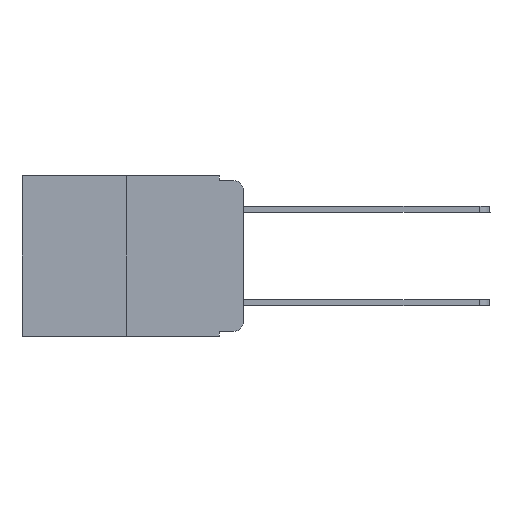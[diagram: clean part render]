
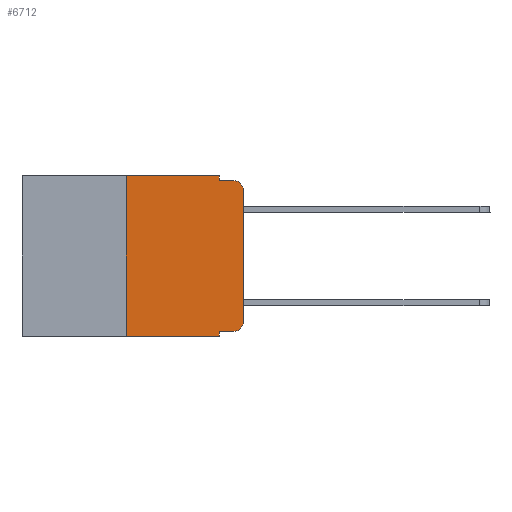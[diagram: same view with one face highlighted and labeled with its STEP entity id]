
A CAD part, left-side view. The second image highlights one B-rep face of the part: STEP entity #6712.
In plain terms, the highlighted planar face has unit normal (-1, 0, 0).
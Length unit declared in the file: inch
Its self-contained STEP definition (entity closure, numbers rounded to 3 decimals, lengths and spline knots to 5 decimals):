
#843 = CARTESIAN_POINT ( 'NONE',  ( 0., 0.25, 0. ) ) ;
#1260 = VECTOR ( 'NONE', #4064, 39.37008 ) ;
#1312 = EDGE_CURVE ( 'NONE', #12646, #7196, #3937, .T. ) ;
#1598 = VECTOR ( 'NONE', #12709, 39.37008 ) ;
#2054 = EDGE_CURVE ( 'NONE', #21031, #15024, #6625, .T. ) ;
#2559 = CARTESIAN_POINT ( 'NONE',  ( 0., 0., -0.03 ) ) ;
#2595 = DIRECTION ( 'NONE',  ( 0., -1., 0. ) ) ;
#2794 = CARTESIAN_POINT ( 'NONE',  ( 0., 0., -0.313 ) ) ;
#3937 = CIRCLE ( 'NONE', #12800, 0.02 ) ;
#4064 = DIRECTION ( 'NONE',  ( 0., -1., 0. ) ) ;
#4126 = ORIENTED_EDGE ( 'NONE', *, *, #8043, .F. ) ;
#4310 = CARTESIAN_POINT ( 'NONE',  ( 0., 0.473, -0.343 ) ) ;
#4584 = VECTOR ( 'NONE', #9415, 39.37008 ) ;
#4660 = DIRECTION ( 'NONE',  ( 0., 0., -1. ) ) ;
#5222 = VERTEX_POINT ( 'NONE', #8206 ) ;
#5336 = VERTEX_POINT ( 'NONE', #10195 ) ;
#5356 = CIRCLE ( 'NONE', #5933, 0.02 ) ;
#5597 = LINE ( 'NONE', #19737, #15118 ) ;
#5824 = DIRECTION ( 'NONE',  ( -1., 0., 0. ) ) ;
#5933 = AXIS2_PLACEMENT_3D ( 'NONE', #21638, #6544, #6464 ) ;
#6302 = DIRECTION ( 'NONE',  ( 1., 0., 0. ) ) ;
#6464 = DIRECTION ( 'NONE',  ( 0., 0., -1. ) ) ;
#6544 = DIRECTION ( 'NONE',  ( -1., 0., 0. ) ) ;
#6625 = LINE ( 'NONE', #4310, #1260 ) ;
#6712 = ADVANCED_FACE ( 'NONE', ( #19662 ), #16188, .F. ) ;
#7117 = CARTESIAN_POINT ( 'NONE',  ( 0., 0.051, -0.01 ) ) ;
#7196 = VERTEX_POINT ( 'NONE', #2794 ) ;
#7393 = VERTEX_POINT ( 'NONE', #14251 ) ;
#7442 = ORIENTED_EDGE ( 'NONE', *, *, #8073, .T. ) ;
#7479 = EDGE_CURVE ( 'NONE', #21050, #5336, #5356, .T. ) ;
#7621 = CARTESIAN_POINT ( 'NONE',  ( 0., 0.051, -0.343 ) ) ;
#7656 = VERTEX_POINT ( 'NONE', #8365 ) ;
#7919 = VECTOR ( 'NONE', #15021, 39.37008 ) ;
#8043 = EDGE_CURVE ( 'NONE', #7656, #5222, #5597, .T. ) ;
#8073 = EDGE_CURVE ( 'NONE', #7393, #12646, #20182, .T. ) ;
#8206 = CARTESIAN_POINT ( 'NONE',  ( 0., 0.051, 0. ) ) ;
#8312 = ORIENTED_EDGE ( 'NONE', *, *, #18660, .F. ) ;
#8330 = EDGE_LOOP ( 'NONE', ( #12256, #11227, #17457, #13143, #4126, #8312, #16956, #19494, #7442, #10292 ) ) ;
#8365 = CARTESIAN_POINT ( 'NONE',  ( 0., 0.25, 0. ) ) ;
#8515 = CARTESIAN_POINT ( 'NONE',  ( 0., 0.051, -0.01 ) ) ;
#9227 = VERTEX_POINT ( 'NONE', #7117 ) ;
#9415 = DIRECTION ( 'NONE',  ( 0., 0., 1. ) ) ;
#10195 = CARTESIAN_POINT ( 'NONE',  ( 0., 0.02, -0.01 ) ) ;
#10292 = ORIENTED_EDGE ( 'NONE', *, *, #1312, .T. ) ;
#11227 = ORIENTED_EDGE ( 'NONE', *, *, #7479, .T. ) ;
#12065 = CARTESIAN_POINT ( 'NONE',  ( 0., 0.051, 0. ) ) ;
#12256 = ORIENTED_EDGE ( 'NONE', *, *, #17833, .T. ) ;
#12416 = LINE ( 'NONE', #8515, #7919 ) ;
#12646 = VERTEX_POINT ( 'NONE', #16381 ) ;
#12709 = DIRECTION ( 'NONE',  ( 0., 0., -1. ) ) ;
#12794 = DIRECTION ( 'NONE',  ( 0., 0., 1. ) ) ;
#12800 = AXIS2_PLACEMENT_3D ( 'NONE', #16087, #5824, #20614 ) ;
#12853 = CARTESIAN_POINT ( 'NONE',  ( 0., 0.051, -0.333 ) ) ;
#12950 = CARTESIAN_POINT ( 'NONE',  ( 0., 0.473, 0. ) ) ;
#13143 = ORIENTED_EDGE ( 'NONE', *, *, #20879, .F. ) ;
#13260 = EDGE_CURVE ( 'NONE', #7393, #15024, #20209, .T. ) ;
#13572 = LINE ( 'NONE', #843, #4584 ) ;
#13980 = CARTESIAN_POINT ( 'NONE',  ( 0., 0., 0. ) ) ;
#14251 = CARTESIAN_POINT ( 'NONE',  ( 0., 0.051, -0.333 ) ) ;
#14387 = CARTESIAN_POINT ( 'NONE',  ( 0., 0.051, 0. ) ) ;
#15021 = DIRECTION ( 'NONE',  ( 0., -1., 0. ) ) ;
#15024 = VERTEX_POINT ( 'NONE', #7621 ) ;
#15118 = VECTOR ( 'NONE', #21387, 39.37008 ) ;
#15380 = DIRECTION ( 'NONE',  ( 0., 0., -1. ) ) ;
#16087 = CARTESIAN_POINT ( 'NONE',  ( 0., 0.02, -0.313 ) ) ;
#16188 = PLANE ( 'NONE',  #19667 ) ;
#16381 = CARTESIAN_POINT ( 'NONE',  ( 0., 0.02, -0.333 ) ) ;
#16956 = ORIENTED_EDGE ( 'NONE', *, *, #2054, .T. ) ;
#17070 = VECTOR ( 'NONE', #12794, 39.37008 ) ;
#17195 = VECTOR ( 'NONE', #15380, 39.37008 ) ;
#17457 = ORIENTED_EDGE ( 'NONE', *, *, #20707, .F. ) ;
#17833 = EDGE_CURVE ( 'NONE', #7196, #21050, #19985, .T. ) ;
#18660 = EDGE_CURVE ( 'NONE', #21031, #7656, #13572, .T. ) ;
#19295 = LINE ( 'NONE', #12065, #17195 ) ;
#19494 = ORIENTED_EDGE ( 'NONE', *, *, #13260, .F. ) ;
#19651 = CARTESIAN_POINT ( 'NONE',  ( 0., 0.25, -0.343 ) ) ;
#19662 = FACE_OUTER_BOUND ( 'NONE', #8330, .T. ) ;
#19667 = AXIS2_PLACEMENT_3D ( 'NONE', #12950, #6302, #4660 ) ;
#19737 = CARTESIAN_POINT ( 'NONE',  ( 0., 0.473, 0. ) ) ;
#19985 = LINE ( 'NONE', #13980, #17070 ) ;
#20182 = LINE ( 'NONE', #12853, #21494 ) ;
#20209 = LINE ( 'NONE', #14387, #1598 ) ;
#20614 = DIRECTION ( 'NONE',  ( 0., 0., -1. ) ) ;
#20707 = EDGE_CURVE ( 'NONE', #9227, #5336, #12416, .T. ) ;
#20879 = EDGE_CURVE ( 'NONE', #5222, #9227, #19295, .T. ) ;
#21031 = VERTEX_POINT ( 'NONE', #19651 ) ;
#21050 = VERTEX_POINT ( 'NONE', #2559 ) ;
#21387 = DIRECTION ( 'NONE',  ( 0., -1., 0. ) ) ;
#21494 = VECTOR ( 'NONE', #2595, 39.37008 ) ;
#21638 = CARTESIAN_POINT ( 'NONE',  ( 0., 0.02, -0.03 ) ) ;
